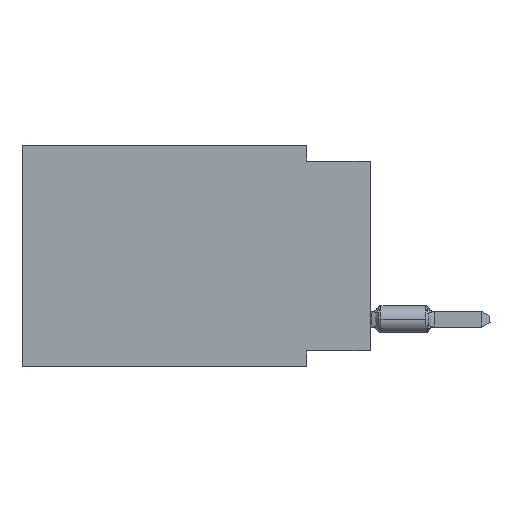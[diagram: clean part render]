
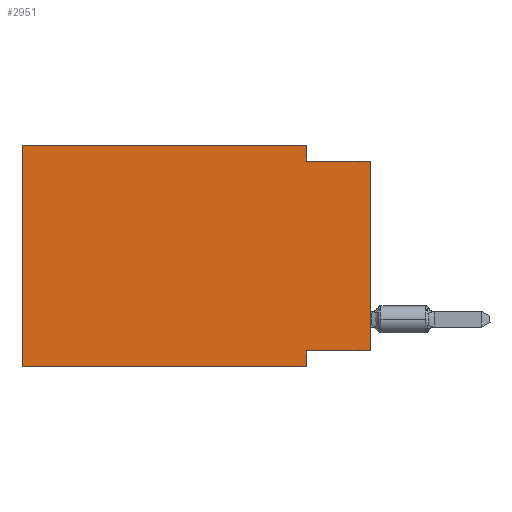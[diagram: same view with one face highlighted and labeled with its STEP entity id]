
A CAD part, left-side view. The second image highlights one B-rep face of the part: STEP entity #2951.
In plain terms, the highlighted planar face has unit normal (-1, 0, 0).
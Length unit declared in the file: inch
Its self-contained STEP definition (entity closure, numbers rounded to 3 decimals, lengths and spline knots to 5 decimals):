
#1157 = ORIENTED_EDGE ( 'NONE', *, *, #6794, .F. ) ;
#1312 = DIRECTION ( 'NONE',  ( 0., -1., 0. ) ) ;
#1390 = CARTESIAN_POINT ( 'NONE',  ( 0., 0.55, 0. ) ) ;
#1665 = LINE ( 'NONE', #18786, #15584 ) ;
#1755 = ORIENTED_EDGE ( 'NONE', *, *, #4308, .F. ) ;
#1953 = CARTESIAN_POINT ( 'NONE',  ( 0., 0.55, 0. ) ) ;
#2001 = EDGE_CURVE ( 'NONE', #18537, #3828, #12649, .T. ) ;
#2028 = ORIENTED_EDGE ( 'NONE', *, *, #4968, .F. ) ;
#2369 = VECTOR ( 'NONE', #17396, 39.37008 ) ;
#2492 = VECTOR ( 'NONE', #14641, 39.37008 ) ;
#2527 = DIRECTION ( 'NONE',  ( 0., -1., 0. ) ) ;
#2951 = ADVANCED_FACE ( 'NONE', ( #3738 ), #18863, .F. ) ;
#3738 = FACE_OUTER_BOUND ( 'NONE', #11420, .T. ) ;
#3784 = CARTESIAN_POINT ( 'NONE',  ( 0., 0.1, -0.35 ) ) ;
#3828 = VERTEX_POINT ( 'NONE', #14917 ) ;
#4308 = EDGE_CURVE ( 'NONE', #8991, #4755, #12306, .T. ) ;
#4447 = VERTEX_POINT ( 'NONE', #8751 ) ;
#4755 = VERTEX_POINT ( 'NONE', #10130 ) ;
#4968 = EDGE_CURVE ( 'NONE', #4755, #3828, #9908, .T. ) ;
#5104 = VERTEX_POINT ( 'NONE', #3784 ) ;
#5113 = LINE ( 'NONE', #1390, #8957 ) ;
#5221 = CARTESIAN_POINT ( 'NONE',  ( 0., 0.55, -0.35 ) ) ;
#5451 = CARTESIAN_POINT ( 'NONE',  ( 0., 0.1, -0.35 ) ) ;
#5809 = EDGE_CURVE ( 'NONE', #9798, #5104, #16595, .T. ) ;
#5839 = CARTESIAN_POINT ( 'NONE',  ( 0., 0., -0.025 ) ) ;
#5945 = ORIENTED_EDGE ( 'NONE', *, *, #2001, .T. ) ;
#6191 = EDGE_CURVE ( 'NONE', #18537, #4447, #1665, .T. ) ;
#6236 = AXIS2_PLACEMENT_3D ( 'NONE', #6482, #8212, #11136 ) ;
#6482 = CARTESIAN_POINT ( 'NONE',  ( 0., 0.55, 0. ) ) ;
#6684 = VECTOR ( 'NONE', #19284, 39.37008 ) ;
#6794 = EDGE_CURVE ( 'NONE', #9798, #17763, #10056, .T. ) ;
#7346 = CARTESIAN_POINT ( 'NONE',  ( 0., 0., 0. ) ) ;
#7477 = CARTESIAN_POINT ( 'NONE',  ( 0., 0.55, 0. ) ) ;
#8143 = ORIENTED_EDGE ( 'NONE', *, *, #13023, .F. ) ;
#8212 = DIRECTION ( 'NONE',  ( 1., 0., 0. ) ) ;
#8751 = CARTESIAN_POINT ( 'NONE',  ( 0., 0.1, -0.325 ) ) ;
#8914 = VECTOR ( 'NONE', #2527, 39.37008 ) ;
#8957 = VECTOR ( 'NONE', #1312, 39.37008 ) ;
#8991 = VERTEX_POINT ( 'NONE', #14812 ) ;
#9798 = VERTEX_POINT ( 'NONE', #14447 ) ;
#9908 = LINE ( 'NONE', #5839, #13010 ) ;
#10056 = LINE ( 'NONE', #1953, #2369 ) ;
#10130 = CARTESIAN_POINT ( 'NONE',  ( 0., 0.1, -0.025 ) ) ;
#10209 = CARTESIAN_POINT ( 'NONE',  ( 0., 0., -0.325 ) ) ;
#10681 = EDGE_CURVE ( 'NONE', #17763, #8991, #5113, .T. ) ;
#11001 = VECTOR ( 'NONE', #19813, 39.37008 ) ;
#11088 = ORIENTED_EDGE ( 'NONE', *, *, #10681, .F. ) ;
#11136 = DIRECTION ( 'NONE',  ( 0., 0., -1. ) ) ;
#11420 = EDGE_LOOP ( 'NONE', ( #5945, #2028, #1755, #11088, #1157, #14951, #8143, #19450 ) ) ;
#12159 = LINE ( 'NONE', #5451, #6684 ) ;
#12306 = LINE ( 'NONE', #14559, #2492 ) ;
#12649 = LINE ( 'NONE', #7346, #11001 ) ;
#13010 = VECTOR ( 'NONE', #13586, 39.37008 ) ;
#13023 = EDGE_CURVE ( 'NONE', #4447, #5104, #12159, .T. ) ;
#13586 = DIRECTION ( 'NONE',  ( 0., -1., 0. ) ) ;
#14447 = CARTESIAN_POINT ( 'NONE',  ( 0., 0.55, -0.35 ) ) ;
#14559 = CARTESIAN_POINT ( 'NONE',  ( 0., 0.1, 0. ) ) ;
#14641 = DIRECTION ( 'NONE',  ( 0., 0., -1. ) ) ;
#14812 = CARTESIAN_POINT ( 'NONE',  ( 0., 0.1, 0. ) ) ;
#14917 = CARTESIAN_POINT ( 'NONE',  ( 0., 0., -0.025 ) ) ;
#14951 = ORIENTED_EDGE ( 'NONE', *, *, #5809, .T. ) ;
#15584 = VECTOR ( 'NONE', #18720, 39.37008 ) ;
#16595 = LINE ( 'NONE', #5221, #8914 ) ;
#17396 = DIRECTION ( 'NONE',  ( 0., 0., 1. ) ) ;
#17763 = VERTEX_POINT ( 'NONE', #7477 ) ;
#18537 = VERTEX_POINT ( 'NONE', #10209 ) ;
#18720 = DIRECTION ( 'NONE',  ( 0., 1., 0. ) ) ;
#18786 = CARTESIAN_POINT ( 'NONE',  ( 0., 0., -0.325 ) ) ;
#18863 = PLANE ( 'NONE',  #6236 ) ;
#19284 = DIRECTION ( 'NONE',  ( 0., 0., -1. ) ) ;
#19450 = ORIENTED_EDGE ( 'NONE', *, *, #6191, .F. ) ;
#19813 = DIRECTION ( 'NONE',  ( 0., 0., 1. ) ) ;
